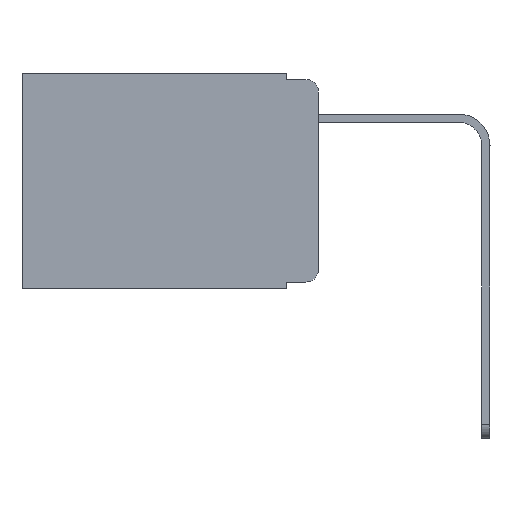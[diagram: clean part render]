
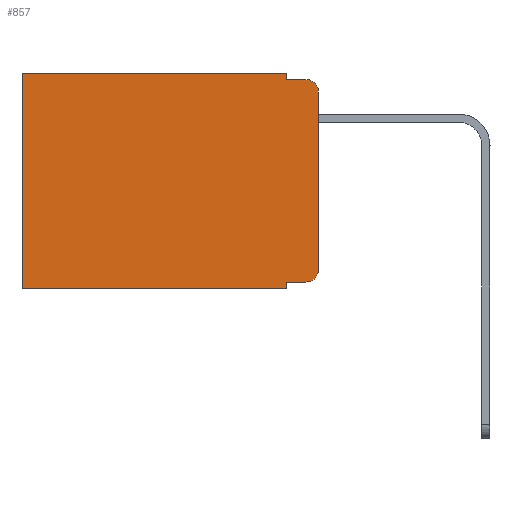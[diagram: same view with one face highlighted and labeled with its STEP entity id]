
A CAD part, left-side view. The second image highlights one B-rep face of the part: STEP entity #857.
In plain terms, the highlighted planar face has unit normal (-1, 0, 0).
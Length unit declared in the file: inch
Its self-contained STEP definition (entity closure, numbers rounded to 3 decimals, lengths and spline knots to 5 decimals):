
#145 = LINE ( 'NONE', #12766, #13359 ) ;
#196 = ORIENTED_EDGE ( 'NONE', *, *, #11582, .T. ) ;
#459 = VERTEX_POINT ( 'NONE', #2098 ) ;
#512 = VERTEX_POINT ( 'NONE', #12600 ) ;
#634 = CARTESIAN_POINT ( 'NONE',  ( 0.298, 0., -0.343 ) ) ;
#857 = ADVANCED_FACE ( 'NONE', ( #3101 ), #2590, .F. ) ;
#913 = EDGE_LOOP ( 'NONE', ( #6827, #1452, #8411, #2394, #12066, #4422, #5392, #9859, #196, #2432 ) ) ;
#1020 = EDGE_CURVE ( 'NONE', #10128, #9678, #10867, .T. ) ;
#1342 = VECTOR ( 'NONE', #1682, 39.37008 ) ;
#1452 = ORIENTED_EDGE ( 'NONE', *, *, #4064, .T. ) ;
#1682 = DIRECTION ( 'NONE',  ( 0., 0., -1. ) ) ;
#2025 = CARTESIAN_POINT ( 'NONE',  ( 0.298, 0., -0.03 ) ) ;
#2098 = CARTESIAN_POINT ( 'NONE',  ( 0.298, 0., -0.313 ) ) ;
#2394 = ORIENTED_EDGE ( 'NONE', *, *, #8572, .F. ) ;
#2432 = ORIENTED_EDGE ( 'NONE', *, *, #5391, .T. ) ;
#2590 = PLANE ( 'NONE',  #14541 ) ;
#2717 = VECTOR ( 'NONE', #3369, 39.37008 ) ;
#2832 = CARTESIAN_POINT ( 'NONE',  ( 0.298, 0., 0. ) ) ;
#2999 = VERTEX_POINT ( 'NONE', #2025 ) ;
#3101 = FACE_OUTER_BOUND ( 'NONE', #913, .T. ) ;
#3369 = DIRECTION ( 'NONE',  ( 0., 1., 0. ) ) ;
#3459 = LINE ( 'NONE', #634, #6080 ) ;
#3520 = DIRECTION ( 'NONE',  ( 0., 0., -1. ) ) ;
#3972 = EDGE_CURVE ( 'NONE', #14466, #512, #3459, .T. ) ;
#4061 = VECTOR ( 'NONE', #11964, 39.37008 ) ;
#4064 = EDGE_CURVE ( 'NONE', #2999, #9678, #12828, .T. ) ;
#4422 = ORIENTED_EDGE ( 'NONE', *, *, #7203, .T. ) ;
#4482 = VERTEX_POINT ( 'NONE', #6624 ) ;
#4498 = DIRECTION ( 'NONE',  ( 0., -1., 0. ) ) ;
#4589 = CARTESIAN_POINT ( 'NONE',  ( 0.298, 0.051, -0.333 ) ) ;
#4986 = VECTOR ( 'NONE', #4498, 39.37008 ) ;
#5038 = AXIS2_PLACEMENT_3D ( 'NONE', #10824, #6374, #5148 ) ;
#5132 = LINE ( 'NONE', #9362, #11370 ) ;
#5148 = DIRECTION ( 'NONE',  ( 0., 0., -1. ) ) ;
#5279 = AXIS2_PLACEMENT_3D ( 'NONE', #10965, #9864, #8695 ) ;
#5391 = EDGE_CURVE ( 'NONE', #8297, #459, #8123, .T. ) ;
#5392 = ORIENTED_EDGE ( 'NONE', *, *, #3972, .F. ) ;
#5640 = CARTESIAN_POINT ( 'NONE',  ( 0.298, 0.473, 0. ) ) ;
#5668 = CARTESIAN_POINT ( 'NONE',  ( 0.298, 0.051, -0.343 ) ) ;
#5791 = CARTESIAN_POINT ( 'NONE',  ( 0.298, 0.473, 0. ) ) ;
#6080 = VECTOR ( 'NONE', #10771, 39.37008 ) ;
#6258 = VECTOR ( 'NONE', #3520, 39.37008 ) ;
#6291 = CARTESIAN_POINT ( 'NONE',  ( 0.298, 0.051, -0.333 ) ) ;
#6374 = DIRECTION ( 'NONE',  ( -1., 0., 0. ) ) ;
#6594 = LINE ( 'NONE', #5640, #6258 ) ;
#6624 = CARTESIAN_POINT ( 'NONE',  ( 0.298, 0.051, 0. ) ) ;
#6827 = ORIENTED_EDGE ( 'NONE', *, *, #13263, .F. ) ;
#6926 = CARTESIAN_POINT ( 'NONE',  ( 0.298, 0.051, 0. ) ) ;
#7203 = EDGE_CURVE ( 'NONE', #12688, #512, #6594, .T. ) ;
#7214 = LINE ( 'NONE', #6926, #1342 ) ;
#7390 = LINE ( 'NONE', #9125, #2717 ) ;
#8123 = CIRCLE ( 'NONE', #5038, 0.02 ) ;
#8297 = VERTEX_POINT ( 'NONE', #8905 ) ;
#8411 = ORIENTED_EDGE ( 'NONE', *, *, #1020, .F. ) ;
#8444 = LINE ( 'NONE', #6291, #4061 ) ;
#8459 = CARTESIAN_POINT ( 'NONE',  ( 0.298, 0.02, -0.01 ) ) ;
#8572 = EDGE_CURVE ( 'NONE', #4482, #10128, #5132, .T. ) ;
#8635 = CARTESIAN_POINT ( 'NONE',  ( 0.298, 0.051, -0.01 ) ) ;
#8695 = DIRECTION ( 'NONE',  ( 0., 0., -1. ) ) ;
#8905 = CARTESIAN_POINT ( 'NONE',  ( 0.298, 0.02, -0.333 ) ) ;
#9125 = CARTESIAN_POINT ( 'NONE',  ( 0.298, 0., 0. ) ) ;
#9362 = CARTESIAN_POINT ( 'NONE',  ( 0.298, 0.051, 0. ) ) ;
#9536 = EDGE_CURVE ( 'NONE', #12552, #14466, #7214, .T. ) ;
#9678 = VERTEX_POINT ( 'NONE', #8459 ) ;
#9859 = ORIENTED_EDGE ( 'NONE', *, *, #9536, .F. ) ;
#9864 = DIRECTION ( 'NONE',  ( -1., 0., 0. ) ) ;
#10128 = VERTEX_POINT ( 'NONE', #8635 ) ;
#10408 = EDGE_CURVE ( 'NONE', #4482, #12688, #7390, .T. ) ;
#10471 = DIRECTION ( 'NONE',  ( 0., 0., -1. ) ) ;
#10712 = DIRECTION ( 'NONE',  ( 1., 0., 0. ) ) ;
#10771 = DIRECTION ( 'NONE',  ( 0., 1., 0. ) ) ;
#10824 = CARTESIAN_POINT ( 'NONE',  ( 0.298, 0.02, -0.313 ) ) ;
#10867 = LINE ( 'NONE', #12419, #4986 ) ;
#10965 = CARTESIAN_POINT ( 'NONE',  ( 0.298, 0.02, -0.03 ) ) ;
#11370 = VECTOR ( 'NONE', #11805, 39.37008 ) ;
#11582 = EDGE_CURVE ( 'NONE', #12552, #8297, #8444, .T. ) ;
#11805 = DIRECTION ( 'NONE',  ( 0., 0., -1. ) ) ;
#11964 = DIRECTION ( 'NONE',  ( 0., -1., 0. ) ) ;
#12066 = ORIENTED_EDGE ( 'NONE', *, *, #10408, .T. ) ;
#12419 = CARTESIAN_POINT ( 'NONE',  ( 0.298, 0.051, -0.01 ) ) ;
#12552 = VERTEX_POINT ( 'NONE', #4589 ) ;
#12600 = CARTESIAN_POINT ( 'NONE',  ( 0.298, 0.473, -0.343 ) ) ;
#12688 = VERTEX_POINT ( 'NONE', #5791 ) ;
#12766 = CARTESIAN_POINT ( 'NONE',  ( 0.298, 0., 0. ) ) ;
#12828 = CIRCLE ( 'NONE', #5279, 0.02 ) ;
#13172 = DIRECTION ( 'NONE',  ( 0., 0., -1. ) ) ;
#13263 = EDGE_CURVE ( 'NONE', #2999, #459, #145, .T. ) ;
#13359 = VECTOR ( 'NONE', #10471, 39.37008 ) ;
#14466 = VERTEX_POINT ( 'NONE', #5668 ) ;
#14541 = AXIS2_PLACEMENT_3D ( 'NONE', #2832, #10712, #13172 ) ;
